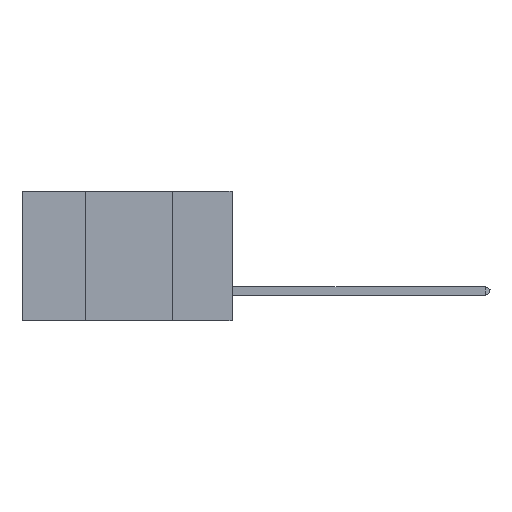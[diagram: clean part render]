
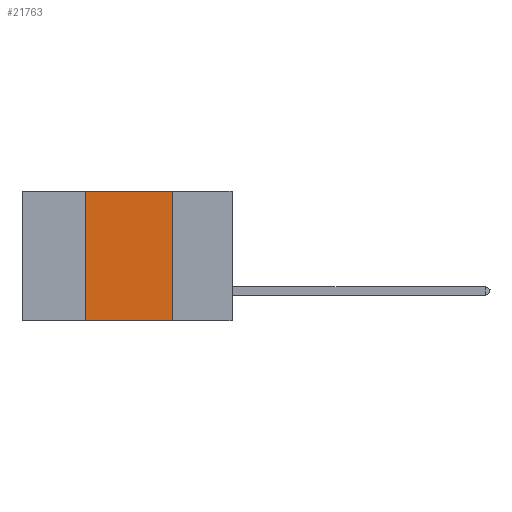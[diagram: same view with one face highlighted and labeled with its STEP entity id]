
A CAD part, left-side view. The second image highlights one B-rep face of the part: STEP entity #21763.
In plain terms, the highlighted planar face has unit normal (-1, 0, 0).
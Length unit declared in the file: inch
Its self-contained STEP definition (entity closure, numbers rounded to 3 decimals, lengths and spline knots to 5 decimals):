
#925 = ORIENTED_EDGE ( 'NONE', *, *, #28444, .F. ) ;
#946 = VECTOR ( 'NONE', #1509, 39.37008 ) ;
#1509 = DIRECTION ( 'NONE',  ( 0., -1., 0. ) ) ;
#1603 = CARTESIAN_POINT ( 'NONE',  ( 0., 0.6, 0. ) ) ;
#1682 = VERTEX_POINT ( 'NONE', #19983 ) ;
#2673 = DIRECTION ( 'NONE',  ( 0., -1., 0. ) ) ;
#2816 = FACE_OUTER_BOUND ( 'NONE', #13654, .T. ) ;
#2979 = LINE ( 'NONE', #33027, #18519 ) ;
#4863 = EDGE_CURVE ( 'NONE', #25726, #1682, #30873, .T. ) ;
#5897 = LINE ( 'NONE', #24409, #10262 ) ;
#6817 = CARTESIAN_POINT ( 'NONE',  ( 0., 0.6, -0.37 ) ) ;
#7258 = DIRECTION ( 'NONE',  ( 0., 0., -1. ) ) ;
#8085 = ORIENTED_EDGE ( 'NONE', *, *, #24114, .T. ) ;
#9442 = VERTEX_POINT ( 'NONE', #30749 ) ;
#10262 = VECTOR ( 'NONE', #19217, 39.37008 ) ;
#11425 = AXIS2_PLACEMENT_3D ( 'NONE', #1603, #18024, #7258 ) ;
#11704 = CARTESIAN_POINT ( 'NONE',  ( 0., 0.42, -0.37 ) ) ;
#12685 = ORIENTED_EDGE ( 'NONE', *, *, #27758, .F. ) ;
#13130 = ORIENTED_EDGE ( 'NONE', *, *, #4863, .F. ) ;
#13654 = EDGE_LOOP ( 'NONE', ( #13130, #12685, #925, #8085 ) ) ;
#15235 = LINE ( 'NONE', #6817, #946 ) ;
#15265 = PLANE ( 'NONE',  #11425 ) ;
#15603 = VERTEX_POINT ( 'NONE', #11704 ) ;
#15694 = VECTOR ( 'NONE', #21897, 39.37008 ) ;
#15977 = CARTESIAN_POINT ( 'NONE',  ( 0., 0.17, 0. ) ) ;
#18024 = DIRECTION ( 'NONE',  ( 1., 0., 0. ) ) ;
#18519 = VECTOR ( 'NONE', #2673, 39.37008 ) ;
#19217 = DIRECTION ( 'NONE',  ( 0., 0., 1. ) ) ;
#19983 = CARTESIAN_POINT ( 'NONE',  ( 0., 0.17, -0.37 ) ) ;
#21763 = ADVANCED_FACE ( 'NONE', ( #2816 ), #15265, .F. ) ;
#21897 = DIRECTION ( 'NONE',  ( 0., 0., -1. ) ) ;
#24114 = EDGE_CURVE ( 'NONE', #15603, #1682, #15235, .T. ) ;
#24409 = CARTESIAN_POINT ( 'NONE',  ( 0., 0.42, 0. ) ) ;
#25726 = VERTEX_POINT ( 'NONE', #33940 ) ;
#27758 = EDGE_CURVE ( 'NONE', #9442, #25726, #2979, .T. ) ;
#28444 = EDGE_CURVE ( 'NONE', #15603, #9442, #5897, .T. ) ;
#30749 = CARTESIAN_POINT ( 'NONE',  ( 0., 0.42, 0. ) ) ;
#30873 = LINE ( 'NONE', #15977, #15694 ) ;
#33027 = CARTESIAN_POINT ( 'NONE',  ( 0., 0.6, 0. ) ) ;
#33940 = CARTESIAN_POINT ( 'NONE',  ( 0., 0.17, 0. ) ) ;
